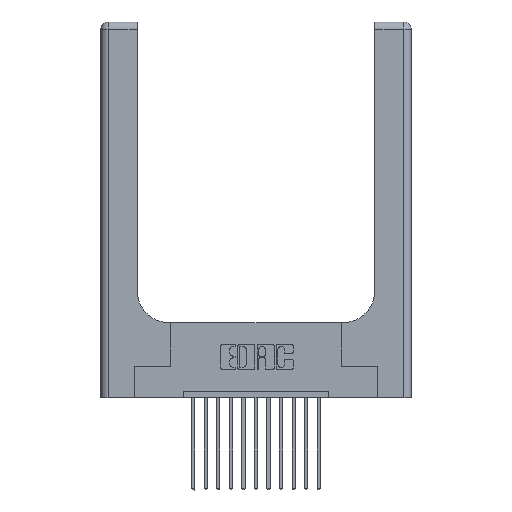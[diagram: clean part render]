
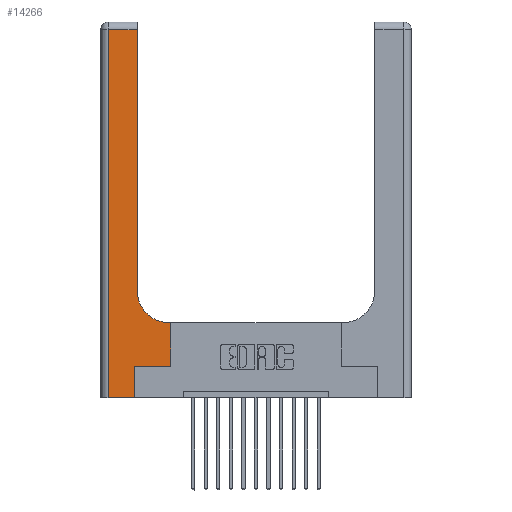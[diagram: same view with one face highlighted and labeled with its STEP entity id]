
A CAD part, top view. The second image highlights one B-rep face of the part: STEP entity #14266.
In plain terms, the highlighted planar face has unit normal (0, 0, 1).
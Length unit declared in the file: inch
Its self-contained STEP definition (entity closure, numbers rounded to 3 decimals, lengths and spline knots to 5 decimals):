
#133 = LINE ( 'NONE', #7847, #2479 ) ;
#548 = VERTEX_POINT ( 'NONE', #15544 ) ;
#665 = DIRECTION ( 'NONE',  ( 1., 0., 0. ) ) ;
#831 = ORIENTED_EDGE ( 'NONE', *, *, #871, .T. ) ;
#871 = EDGE_CURVE ( 'NONE', #14343, #10290, #2632, .T. ) ;
#1245 = EDGE_CURVE ( 'NONE', #4529, #10833, #9198, .T. ) ;
#1382 = CARTESIAN_POINT ( 'NONE',  ( 0.06, 2.94, 0.37 ) ) ;
#1711 = ORIENTED_EDGE ( 'NONE', *, *, #3010, .T. ) ;
#1726 = AXIS2_PLACEMENT_3D ( 'NONE', #12804, #16796, #3131 ) ;
#1991 = PLANE ( 'NONE',  #1726 ) ;
#2056 = ORIENTED_EDGE ( 'NONE', *, *, #5760, .T. ) ;
#2479 = VECTOR ( 'NONE', #6429, 39.37008 ) ;
#2632 = CIRCLE ( 'NONE', #16905, 0.25 ) ;
#2690 = VECTOR ( 'NONE', #13173, 39.37008 ) ;
#2784 = DIRECTION ( 'NONE',  ( -1., 0., 0. ) ) ;
#2995 = CARTESIAN_POINT ( 'NONE',  ( 0.5585, 0.25, 0.37 ) ) ;
#3010 = EDGE_CURVE ( 'NONE', #11362, #14343, #15358, .T. ) ;
#3131 = DIRECTION ( 'NONE',  ( -1., 0., 0. ) ) ;
#3926 = LINE ( 'NONE', #4091, #14388 ) ;
#3927 = CARTESIAN_POINT ( 'NONE',  ( 0.269, 0., 0.37 ) ) ;
#4091 = CARTESIAN_POINT ( 'NONE',  ( 0., 2.94, 0.37 ) ) ;
#4383 = VERTEX_POINT ( 'NONE', #2995 ) ;
#4404 = CARTESIAN_POINT ( 'NONE',  ( 0.269, 0.25, 0.37 ) ) ;
#4425 = CARTESIAN_POINT ( 'NONE',  ( 0.2915, 0.85, 0.37 ) ) ;
#4529 = VERTEX_POINT ( 'NONE', #13553 ) ;
#4543 = CARTESIAN_POINT ( 'NONE',  ( 0.5585, 0.6, 0.37 ) ) ;
#4766 = VECTOR ( 'NONE', #8891, 39.37008 ) ;
#4860 = CARTESIAN_POINT ( 'NONE',  ( 0.5415, 0.6, 0.37 ) ) ;
#4990 = CARTESIAN_POINT ( 'NONE',  ( 0.5415, 0.85, 0.37 ) ) ;
#5705 = CARTESIAN_POINT ( 'NONE',  ( 0.2915, 0.6, 0.37 ) ) ;
#5760 = EDGE_CURVE ( 'NONE', #4383, #11362, #10372, .T. ) ;
#5838 = ORIENTED_EDGE ( 'NONE', *, *, #12608, .T. ) ;
#6126 = EDGE_CURVE ( 'NONE', #10290, #12965, #7772, .T. ) ;
#6198 = VECTOR ( 'NONE', #9722, 39.37008 ) ;
#6429 = DIRECTION ( 'NONE',  ( 0., -1., 0. ) ) ;
#7268 = DIRECTION ( 'NONE',  ( 0., 0., -1. ) ) ;
#7413 = CARTESIAN_POINT ( 'NONE',  ( 0.2915, 3., 0.37 ) ) ;
#7772 = LINE ( 'NONE', #7413, #10561 ) ;
#7847 = CARTESIAN_POINT ( 'NONE',  ( 0.06, 3., 0.37 ) ) ;
#7920 = CARTESIAN_POINT ( 'NONE',  ( 0.2915, 2.94, 0.37 ) ) ;
#8155 = ORIENTED_EDGE ( 'NONE', *, *, #1245, .T. ) ;
#8420 = DIRECTION ( 'NONE',  ( -1., 0., 0. ) ) ;
#8891 = DIRECTION ( 'NONE',  ( 0., 1., 0. ) ) ;
#8915 = ORIENTED_EDGE ( 'NONE', *, *, #11241, .T. ) ;
#9163 = CARTESIAN_POINT ( 'NONE',  ( 0.5585, 0.25, 0.37 ) ) ;
#9198 = LINE ( 'NONE', #3927, #4766 ) ;
#9564 = ORIENTED_EDGE ( 'NONE', *, *, #6126, .T. ) ;
#9722 = DIRECTION ( 'NONE',  ( 1., 0., 0. ) ) ;
#10069 = EDGE_CURVE ( 'NONE', #16216, #548, #133, .T. ) ;
#10290 = VERTEX_POINT ( 'NONE', #4425 ) ;
#10372 = LINE ( 'NONE', #9163, #2690 ) ;
#10561 = VECTOR ( 'NONE', #10634, 39.37008 ) ;
#10634 = DIRECTION ( 'NONE',  ( 0., 1., 0. ) ) ;
#10817 = CARTESIAN_POINT ( 'NONE',  ( 0., 0., 0.37 ) ) ;
#10833 = VERTEX_POINT ( 'NONE', #4404 ) ;
#11241 = EDGE_CURVE ( 'NONE', #12965, #16216, #3926, .T. ) ;
#11362 = VERTEX_POINT ( 'NONE', #4543 ) ;
#11727 = VECTOR ( 'NONE', #8420, 39.37008 ) ;
#11957 = ORIENTED_EDGE ( 'NONE', *, *, #10069, .T. ) ;
#12398 = EDGE_CURVE ( 'NONE', #548, #4529, #15843, .T. ) ;
#12475 = FACE_OUTER_BOUND ( 'NONE', #14540, .T. ) ;
#12608 = EDGE_CURVE ( 'NONE', #10833, #4383, #16243, .T. ) ;
#12804 = CARTESIAN_POINT ( 'NONE',  ( 0., 3., 0.37 ) ) ;
#12949 = ORIENTED_EDGE ( 'NONE', *, *, #12398, .T. ) ;
#12965 = VERTEX_POINT ( 'NONE', #7920 ) ;
#13173 = DIRECTION ( 'NONE',  ( 0., 1., 0. ) ) ;
#13553 = CARTESIAN_POINT ( 'NONE',  ( 0.269, 0., 0.37 ) ) ;
#14266 = ADVANCED_FACE ( 'NONE', ( #12475 ), #1991, .F. ) ;
#14343 = VERTEX_POINT ( 'NONE', #4860 ) ;
#14388 = VECTOR ( 'NONE', #2784, 39.37008 ) ;
#14540 = EDGE_LOOP ( 'NONE', ( #9564, #8915, #11957, #12949, #8155, #5838, #2056, #1711, #831 ) ) ;
#15358 = LINE ( 'NONE', #5705, #11727 ) ;
#15544 = CARTESIAN_POINT ( 'NONE',  ( 0.06, 0., 0.37 ) ) ;
#15622 = CARTESIAN_POINT ( 'NONE',  ( 0.269, 0.25, 0.37 ) ) ;
#15843 = LINE ( 'NONE', #10817, #6198 ) ;
#16023 = DIRECTION ( 'NONE',  ( 1., 0., 0. ) ) ;
#16216 = VERTEX_POINT ( 'NONE', #1382 ) ;
#16243 = LINE ( 'NONE', #15622, #17522 ) ;
#16796 = DIRECTION ( 'NONE',  ( 0., 0., -1. ) ) ;
#16905 = AXIS2_PLACEMENT_3D ( 'NONE', #4990, #7268, #16023 ) ;
#17522 = VECTOR ( 'NONE', #665, 39.37008 ) ;
